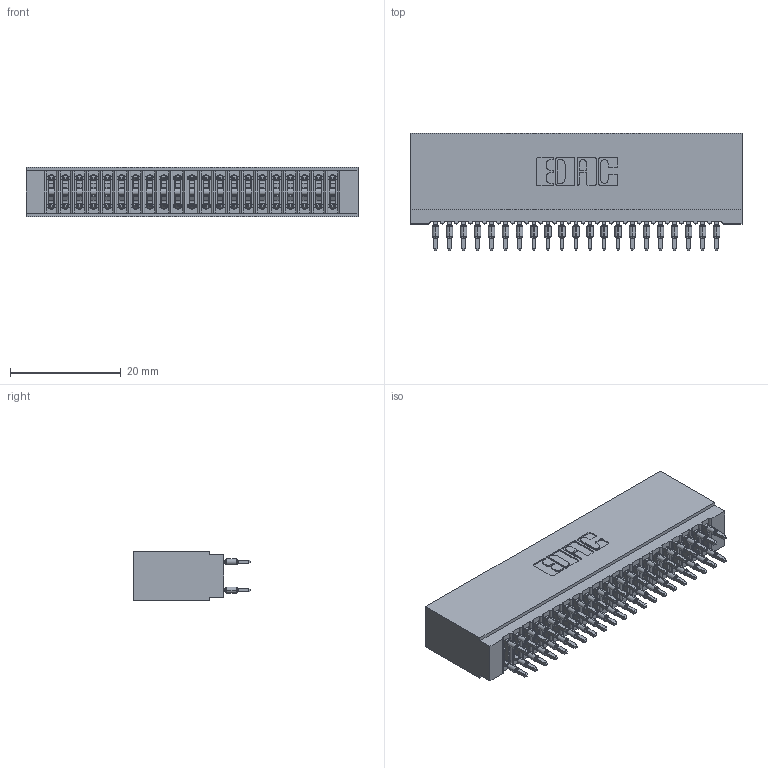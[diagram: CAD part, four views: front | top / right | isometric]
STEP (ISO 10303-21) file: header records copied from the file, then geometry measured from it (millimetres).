
FILE_DESCRIPTION (( 'STEP AP203' ), '1' );
FILE_NAME ('745-042-560-201.STEP', '2026-02-26T17:45:32', ( '' ), ( '' ), 'SwSTEP 2.0', 'SolidWorks 2023', '' );
FILE_SCHEMA (( 'CONFIG_CONTROL_DESIGN' ));
Length unit declared in the file: millimetre
Products named in the file (3): 745-292-001_560; 745-042-560-201; 745 Part_Insulator Option - 01
Assembly tree (43 placements, depth 2):
  745-042-560-201
    745 Part_Insulator Option - 01
    745-292-001_560  x42
Bounding box: 59.94 x 21.22 x 8.89 mm (x, y, z)
Volume: 5681.1 mm3; surface area: 11725 mm2
Topology: 43 solids, 43 shells, 4232 faces, 11577 edges, 7354 vertices
Faces by surface type: plane 2197, cylinder 943, bspline 840, torus 252
Entity records: 38544 total; most frequent: CARTESIAN_POINT 7197, ORIENTED_EDGE 6590, DIRECTION 5779, EDGE_CURVE 3295, LINE 2979, VECTOR 2979, VERTEX_POINT 2106, AXIS2_PLACEMENT_3D 1400
